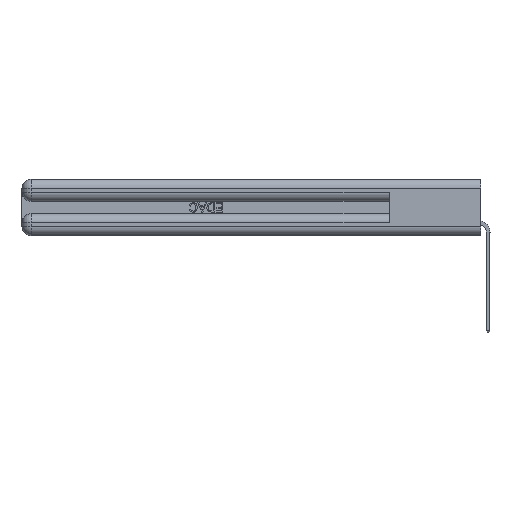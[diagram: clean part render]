
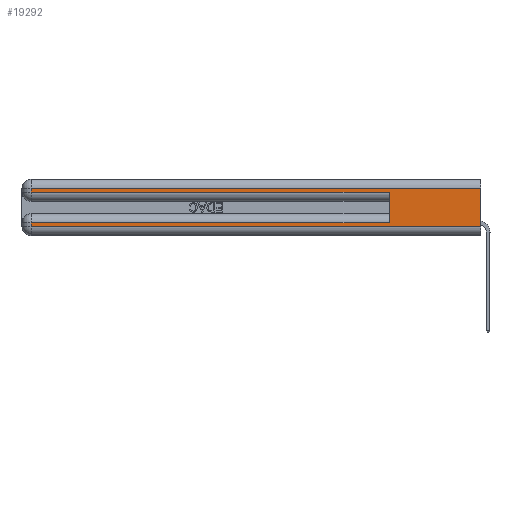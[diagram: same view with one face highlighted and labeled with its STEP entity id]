
A CAD part, left-side view. The second image highlights one B-rep face of the part: STEP entity #19292.
In plain terms, the highlighted planar face has unit normal (-1, 0, 0).
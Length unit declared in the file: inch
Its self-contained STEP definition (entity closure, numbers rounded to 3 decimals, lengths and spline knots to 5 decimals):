
#24 = ORIENTED_EDGE ( 'NONE', *, *, #3048, .T. ) ;
#404 = DIRECTION ( 'NONE',  ( 0., 0., -1. ) ) ;
#874 = FACE_OUTER_BOUND ( 'NONE', #6461, .T. ) ;
#3048 = EDGE_CURVE ( 'NONE', #15598, #14932, #46191, .T. ) ;
#4268 = LINE ( 'NONE', #14482, #37728 ) ;
#6191 = DIRECTION ( 'NONE',  ( 1., 0., 0. ) ) ;
#6461 = EDGE_LOOP ( 'NONE', ( #24490, #24185, #19125, #24256, #38261, #44539, #24, #6681 ) ) ;
#6681 = ORIENTED_EDGE ( 'NONE', *, *, #28368, .T. ) ;
#7659 = EDGE_CURVE ( 'NONE', #33384, #15598, #39185, .T. ) ;
#11453 = CARTESIAN_POINT ( 'NONE',  ( 0., 0., 0.31 ) ) ;
#12336 = VECTOR ( 'NONE', #22157, 39.37008 ) ;
#12565 = VECTOR ( 'NONE', #404, 39.37008 ) ;
#13523 = VERTEX_POINT ( 'NONE', #43515 ) ;
#14390 = CARTESIAN_POINT ( 'NONE',  ( 0., 0.6, 0.085 ) ) ;
#14482 = CARTESIAN_POINT ( 'NONE',  ( 0., 0., 0.06 ) ) ;
#14867 = VECTOR ( 'NONE', #23864, 39.37008 ) ;
#14932 = VERTEX_POINT ( 'NONE', #43155 ) ;
#15598 = VERTEX_POINT ( 'NONE', #27122 ) ;
#16279 = CARTESIAN_POINT ( 'NONE',  ( 0., 2.94, 0.37 ) ) ;
#17348 = CARTESIAN_POINT ( 'NONE',  ( 0., 0.6, 0.285 ) ) ;
#17804 = LINE ( 'NONE', #11453, #42204 ) ;
#18506 = CARTESIAN_POINT ( 'NONE',  ( 0., 0., 0.285 ) ) ;
#18572 = CARTESIAN_POINT ( 'NONE',  ( 0., 2.94, 0.37 ) ) ;
#19125 = ORIENTED_EDGE ( 'NONE', *, *, #26424, .T. ) ;
#19292 = ADVANCED_FACE ( 'NONE', ( #874 ), #32707, .F. ) ;
#20056 = CARTESIAN_POINT ( 'NONE',  ( 0., 0., 0.31 ) ) ;
#21278 = DIRECTION ( 'NONE',  ( 0., 1., 0. ) ) ;
#21533 = CARTESIAN_POINT ( 'NONE',  ( 0., 0., 0.37 ) ) ;
#22157 = DIRECTION ( 'NONE',  ( 0., -1., 0. ) ) ;
#22320 = EDGE_CURVE ( 'NONE', #30541, #39934, #32746, .T. ) ;
#23796 = CARTESIAN_POINT ( 'NONE',  ( 0., 0.6, 0.145 ) ) ;
#23864 = DIRECTION ( 'NONE',  ( 0., 0., -1. ) ) ;
#24090 = VECTOR ( 'NONE', #31038, 39.37008 ) ;
#24185 = ORIENTED_EDGE ( 'NONE', *, *, #40655, .T. ) ;
#24256 = ORIENTED_EDGE ( 'NONE', *, *, #39598, .T. ) ;
#24490 = ORIENTED_EDGE ( 'NONE', *, *, #22320, .F. ) ;
#25257 = AXIS2_PLACEMENT_3D ( 'NONE', #21533, #6191, #28511 ) ;
#25483 = CARTESIAN_POINT ( 'NONE',  ( 0., 2.94, 0.285 ) ) ;
#26424 = EDGE_CURVE ( 'NONE', #13523, #43704, #33518, .T. ) ;
#27122 = CARTESIAN_POINT ( 'NONE',  ( 0., 2.94, 0.085 ) ) ;
#28368 = EDGE_CURVE ( 'NONE', #14932, #39934, #4268, .T. ) ;
#28477 = VECTOR ( 'NONE', #21278, 39.37008 ) ;
#28511 = DIRECTION ( 'NONE',  ( 0., 0., -1. ) ) ;
#29673 = VECTOR ( 'NONE', #46786, 39.37008 ) ;
#30541 = VERTEX_POINT ( 'NONE', #20056 ) ;
#30605 = EDGE_CURVE ( 'NONE', #33384, #39591, #44584, .T. ) ;
#31038 = DIRECTION ( 'NONE',  ( 0., 0., -1. ) ) ;
#32617 = CARTESIAN_POINT ( 'NONE',  ( 0., 0., 0.085 ) ) ;
#32707 = PLANE ( 'NONE',  #25257 ) ;
#32746 = LINE ( 'NONE', #34869, #14867 ) ;
#33384 = VERTEX_POINT ( 'NONE', #14390 ) ;
#33468 = DIRECTION ( 'NONE',  ( 0., -1., 0. ) ) ;
#33518 = LINE ( 'NONE', #18572, #12565 ) ;
#34869 = CARTESIAN_POINT ( 'NONE',  ( 0., 0., 0.37 ) ) ;
#37728 = VECTOR ( 'NONE', #33468, 39.37008 ) ;
#38261 = ORIENTED_EDGE ( 'NONE', *, *, #30605, .F. ) ;
#39185 = LINE ( 'NONE', #32617, #28477 ) ;
#39419 = DIRECTION ( 'NONE',  ( 0., 1., 0. ) ) ;
#39591 = VERTEX_POINT ( 'NONE', #17348 ) ;
#39598 = EDGE_CURVE ( 'NONE', #43704, #39591, #39803, .T. ) ;
#39803 = LINE ( 'NONE', #18506, #12336 ) ;
#39934 = VERTEX_POINT ( 'NONE', #45838 ) ;
#40655 = EDGE_CURVE ( 'NONE', #30541, #13523, #17804, .T. ) ;
#42204 = VECTOR ( 'NONE', #39419, 39.37008 ) ;
#43155 = CARTESIAN_POINT ( 'NONE',  ( 0., 2.94, 0.06 ) ) ;
#43515 = CARTESIAN_POINT ( 'NONE',  ( 0., 2.94, 0.31 ) ) ;
#43704 = VERTEX_POINT ( 'NONE', #25483 ) ;
#44539 = ORIENTED_EDGE ( 'NONE', *, *, #7659, .T. ) ;
#44584 = LINE ( 'NONE', #23796, #29673 ) ;
#45838 = CARTESIAN_POINT ( 'NONE',  ( 0., 0., 0.06 ) ) ;
#46191 = LINE ( 'NONE', #16279, #24090 ) ;
#46786 = DIRECTION ( 'NONE',  ( 0., 0., 1. ) ) ;
